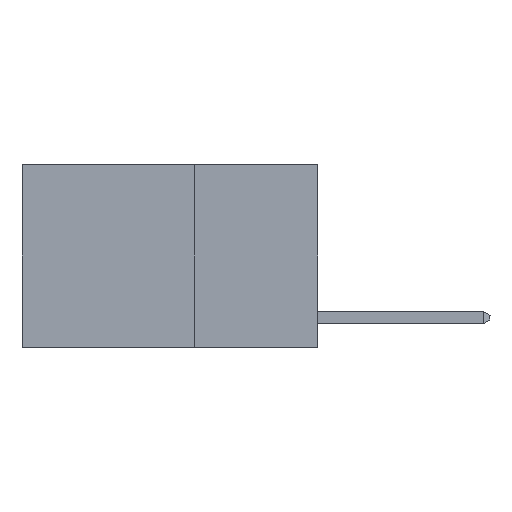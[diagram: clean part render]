
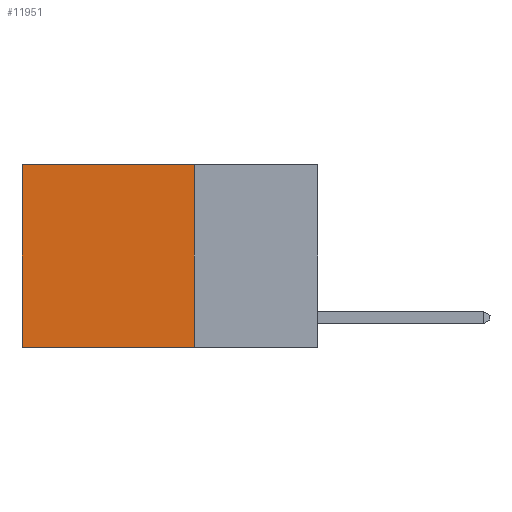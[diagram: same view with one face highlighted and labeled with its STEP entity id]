
A CAD part, left-side view. The second image highlights one B-rep face of the part: STEP entity #11951.
In plain terms, the highlighted planar face has unit normal (-1, 0, 0).
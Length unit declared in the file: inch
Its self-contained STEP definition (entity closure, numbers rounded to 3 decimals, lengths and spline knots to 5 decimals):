
#374 = CARTESIAN_POINT ( 'NONE',  ( 0.2625, 0.25, -0.37 ) ) ;
#1036 = CARTESIAN_POINT ( 'NONE',  ( 0.2625, 0.25, -0.37 ) ) ;
#1311 = LINE ( 'NONE', #11040, #6257 ) ;
#1780 = VERTEX_POINT ( 'NONE', #19056 ) ;
#1956 = DIRECTION ( 'NONE',  ( 0., 1., 0. ) ) ;
#2736 = EDGE_CURVE ( 'NONE', #8932, #4660, #1311, .T. ) ;
#3867 = FACE_OUTER_BOUND ( 'NONE', #9005, .T. ) ;
#3982 = PLANE ( 'NONE',  #10228 ) ;
#4631 = ORIENTED_EDGE ( 'NONE', *, *, #2736, .T. ) ;
#4660 = VERTEX_POINT ( 'NONE', #6943 ) ;
#5582 = DIRECTION ( 'NONE',  ( 1., 0., 0. ) ) ;
#6257 = VECTOR ( 'NONE', #17831, 39.37008 ) ;
#6650 = EDGE_CURVE ( 'NONE', #1780, #7860, #13341, .T. ) ;
#6943 = CARTESIAN_POINT ( 'NONE',  ( 0.2625, 0.6, -0.37 ) ) ;
#7575 = VECTOR ( 'NONE', #1956, 39.37008 ) ;
#7860 = VERTEX_POINT ( 'NONE', #374 ) ;
#8932 = VERTEX_POINT ( 'NONE', #16167 ) ;
#9005 = EDGE_LOOP ( 'NONE', ( #4631, #14931, #11024, #18702 ) ) ;
#9191 = VECTOR ( 'NONE', #17951, 39.37008 ) ;
#10228 = AXIS2_PLACEMENT_3D ( 'NONE', #10409, #5582, #16988 ) ;
#10302 = CARTESIAN_POINT ( 'NONE',  ( 0.2625, 0.25, 0. ) ) ;
#10409 = CARTESIAN_POINT ( 'NONE',  ( 0.2625, 0.25, 0. ) ) ;
#11024 = ORIENTED_EDGE ( 'NONE', *, *, #6650, .F. ) ;
#11040 = CARTESIAN_POINT ( 'NONE',  ( 0.2625, 0.6, 0. ) ) ;
#11377 = LINE ( 'NONE', #1036, #9191 ) ;
#11661 = EDGE_CURVE ( 'NONE', #7860, #4660, #11377, .T. ) ;
#11951 = ADVANCED_FACE ( 'NONE', ( #3867 ), #3982, .F. ) ;
#13335 = CARTESIAN_POINT ( 'NONE',  ( 0.2625, 0.25, 0. ) ) ;
#13341 = LINE ( 'NONE', #10302, #19101 ) ;
#14831 = LINE ( 'NONE', #13335, #7575 ) ;
#14931 = ORIENTED_EDGE ( 'NONE', *, *, #11661, .F. ) ;
#16167 = CARTESIAN_POINT ( 'NONE',  ( 0.2625, 0.6, 0. ) ) ;
#16564 = DIRECTION ( 'NONE',  ( 0., 0., -1. ) ) ;
#16988 = DIRECTION ( 'NONE',  ( 0., 0., -1. ) ) ;
#17831 = DIRECTION ( 'NONE',  ( 0., 0., -1. ) ) ;
#17951 = DIRECTION ( 'NONE',  ( 0., 1., 0. ) ) ;
#18702 = ORIENTED_EDGE ( 'NONE', *, *, #18848, .T. ) ;
#18848 = EDGE_CURVE ( 'NONE', #1780, #8932, #14831, .T. ) ;
#19056 = CARTESIAN_POINT ( 'NONE',  ( 0.2625, 0.25, 0. ) ) ;
#19101 = VECTOR ( 'NONE', #16564, 39.37008 ) ;
